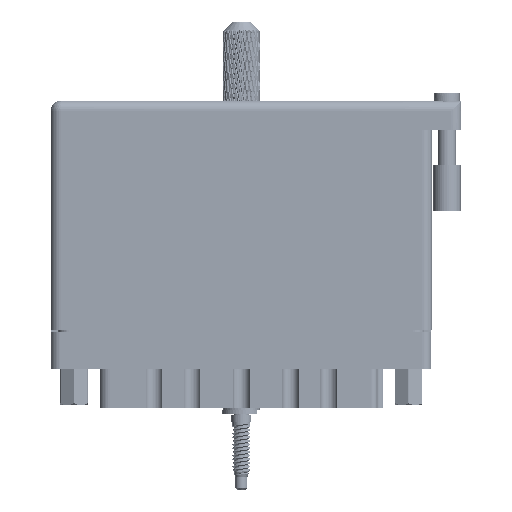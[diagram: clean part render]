
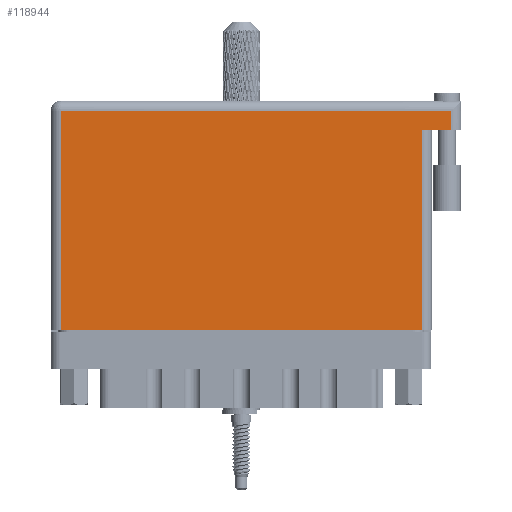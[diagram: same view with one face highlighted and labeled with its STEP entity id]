
A CAD part, front view. The second image highlights one B-rep face of the part: STEP entity #118944.
In plain terms, the highlighted face is planar.
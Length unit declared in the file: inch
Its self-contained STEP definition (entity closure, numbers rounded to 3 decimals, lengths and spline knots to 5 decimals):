
#3765 = ORIENTED_EDGE ( 'NONE', *, *, #83335, .T. ) ;
#5700 = DIRECTION ( 'NONE',  ( 0., 1., 0. ) ) ;
#7566 = CARTESIAN_POINT ( 'NONE',  ( 0., 1.566, 0. ) ) ;
#9259 = DIRECTION ( 'NONE',  ( 0., 0., -1. ) ) ;
#9425 = EDGE_CURVE ( 'NONE', #69986, #23565, #85304, .T. ) ;
#9634 = FACE_OUTER_BOUND ( 'NONE', #27038, .T. ) ;
#10812 = VERTEX_POINT ( 'NONE', #27057 ) ;
#16551 = CARTESIAN_POINT ( 'NONE',  ( 0.07, 0., 0. ) ) ;
#21807 = DIRECTION ( 'NONE',  ( 0., 1., 0. ) ) ;
#23565 = VERTEX_POINT ( 'NONE', #87203 ) ;
#27038 = EDGE_LOOP ( 'NONE', ( #94679, #116171, #32234, #84697, #94489, #3765 ) ) ;
#27057 = CARTESIAN_POINT ( 'NONE',  ( 2.53, 1.369, 0. ) ) ;
#30894 = LINE ( 'NONE', #45840, #91071 ) ;
#32234 = ORIENTED_EDGE ( 'NONE', *, *, #122151, .F. ) ;
#32317 = CARTESIAN_POINT ( 'NONE',  ( 0., 0., 0. ) ) ;
#34751 = AXIS2_PLACEMENT_3D ( 'NONE', #7566, #9259, #117678 ) ;
#45840 = CARTESIAN_POINT ( 'NONE',  ( 2.53, 1.369, 0. ) ) ;
#48031 = EDGE_CURVE ( 'NONE', #49629, #10812, #30894, .T. ) ;
#48536 = DIRECTION ( 'NONE',  ( -1., 0., 0. ) ) ;
#49629 = VERTEX_POINT ( 'NONE', #117229 ) ;
#51324 = CARTESIAN_POINT ( 'NONE',  ( 0.07, 0., 0. ) ) ;
#53280 = CARTESIAN_POINT ( 'NONE',  ( 2.73, 1.496, 0. ) ) ;
#54124 = DIRECTION ( 'NONE',  ( -1., 0., 0. ) ) ;
#56228 = DIRECTION ( 'NONE',  ( 0., -1., 0. ) ) ;
#59037 = VECTOR ( 'NONE', #48536, 39.37008 ) ;
#65426 = VECTOR ( 'NONE', #92739, 39.37008 ) ;
#66484 = VERTEX_POINT ( 'NONE', #51324 ) ;
#67692 = VECTOR ( 'NONE', #21807, 39.37008 ) ;
#69986 = VERTEX_POINT ( 'NONE', #53280 ) ;
#72178 = CARTESIAN_POINT ( 'NONE',  ( 2.8, 1.369, 0. ) ) ;
#75435 = VECTOR ( 'NONE', #54124, 39.37008 ) ;
#80839 = CARTESIAN_POINT ( 'NONE',  ( 2.73, 1.566, 0. ) ) ;
#83335 = EDGE_CURVE ( 'NONE', #23565, #66484, #103829, .T. ) ;
#84697 = ORIENTED_EDGE ( 'NONE', *, *, #99134, .T. ) ;
#85235 = PLANE ( 'NONE',  #34751 ) ;
#85304 = LINE ( 'NONE', #97831, #59037 ) ;
#87203 = CARTESIAN_POINT ( 'NONE',  ( 0.07, 1.496, 0. ) ) ;
#91071 = VECTOR ( 'NONE', #5700, 39.37008 ) ;
#92739 = DIRECTION ( 'NONE',  ( 1., 0., 0. ) ) ;
#93217 = EDGE_CURVE ( 'NONE', #66484, #49629, #96386, .T. ) ;
#94489 = ORIENTED_EDGE ( 'NONE', *, *, #9425, .T. ) ;
#94529 = VECTOR ( 'NONE', #56228, 39.37008 ) ;
#94679 = ORIENTED_EDGE ( 'NONE', *, *, #93217, .T. ) ;
#96386 = LINE ( 'NONE', #32317, #65426 ) ;
#97831 = CARTESIAN_POINT ( 'NONE',  ( 0., 1.496, 0. ) ) ;
#99134 = EDGE_CURVE ( 'NONE', #104858, #69986, #114177, .T. ) ;
#103829 = LINE ( 'NONE', #16551, #94529 ) ;
#104858 = VERTEX_POINT ( 'NONE', #111500 ) ;
#111500 = CARTESIAN_POINT ( 'NONE',  ( 2.73, 1.369, 0. ) ) ;
#114177 = LINE ( 'NONE', #80839, #67692 ) ;
#116171 = ORIENTED_EDGE ( 'NONE', *, *, #48031, .T. ) ;
#117229 = CARTESIAN_POINT ( 'NONE',  ( 2.53, 0., 0. ) ) ;
#117678 = DIRECTION ( 'NONE',  ( -1., 0., 0. ) ) ;
#118944 = ADVANCED_FACE ( 'NONE', ( #9634 ), #85235, .F. ) ;
#121873 = LINE ( 'NONE', #72178, #75435 ) ;
#122151 = EDGE_CURVE ( 'NONE', #104858, #10812, #121873, .T. ) ;
